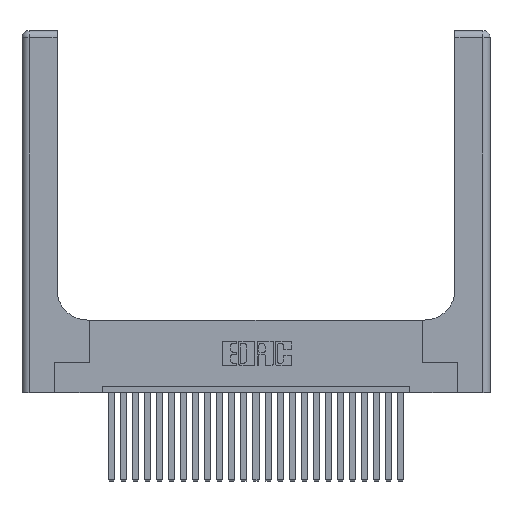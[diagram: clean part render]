
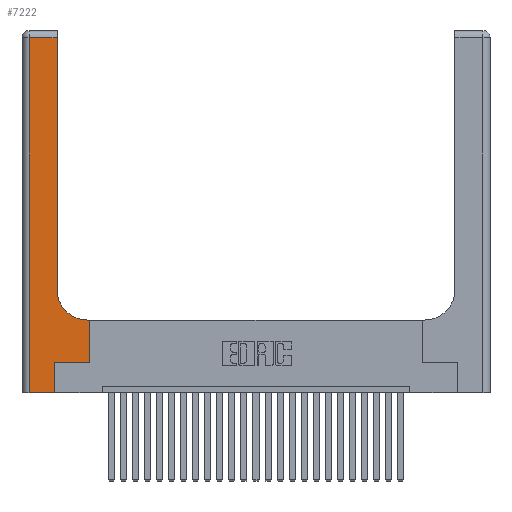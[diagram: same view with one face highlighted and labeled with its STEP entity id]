
A CAD part, top view. The second image highlights one B-rep face of the part: STEP entity #7222.
In plain terms, the highlighted planar face has unit normal (0, 0, 1).
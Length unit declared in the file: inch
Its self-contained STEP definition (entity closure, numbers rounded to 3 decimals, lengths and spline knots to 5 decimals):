
#53 = VERTEX_POINT ( 'NONE', #1612 ) ;
#74 = AXIS2_PLACEMENT_3D ( 'NONE', #4437, #18707, #6820 ) ;
#251 = CARTESIAN_POINT ( 'NONE',  ( 0.269, 0., 0.37 ) ) ;
#652 = VECTOR ( 'NONE', #22442, 39.37008 ) ;
#1354 = CARTESIAN_POINT ( 'NONE',  ( 0.269, 0.25, 0.37 ) ) ;
#1612 = CARTESIAN_POINT ( 'NONE',  ( 0.06, 2.94, 0.37 ) ) ;
#2027 = LINE ( 'NONE', #4778, #13988 ) ;
#2198 = DIRECTION ( 'NONE',  ( 0., 1., 0. ) ) ;
#2358 = VECTOR ( 'NONE', #20729, 39.37008 ) ;
#2909 = VERTEX_POINT ( 'NONE', #25321 ) ;
#2932 = LINE ( 'NONE', #18457, #23054 ) ;
#3047 = ORIENTED_EDGE ( 'NONE', *, *, #14848, .T. ) ;
#3260 = DIRECTION ( 'NONE',  ( 0., 0., -1. ) ) ;
#3556 = ORIENTED_EDGE ( 'NONE', *, *, #8674, .T. ) ;
#4031 = VERTEX_POINT ( 'NONE', #25972 ) ;
#4101 = ORIENTED_EDGE ( 'NONE', *, *, #18121, .T. ) ;
#4437 = CARTESIAN_POINT ( 'NONE',  ( 0.5415, 0.85, 0.37 ) ) ;
#4513 = ORIENTED_EDGE ( 'NONE', *, *, #19888, .T. ) ;
#4575 = ORIENTED_EDGE ( 'NONE', *, *, #22186, .T. ) ;
#4778 = CARTESIAN_POINT ( 'NONE',  ( 0.5585, 0.25, 0.37 ) ) ;
#4822 = CARTESIAN_POINT ( 'NONE',  ( 0.269, 0.25, 0.37 ) ) ;
#5112 = DIRECTION ( 'NONE',  ( -1., 0., 0. ) ) ;
#5388 = VERTEX_POINT ( 'NONE', #13021 ) ;
#5740 = ORIENTED_EDGE ( 'NONE', *, *, #19555, .T. ) ;
#5944 = CIRCLE ( 'NONE', #74, 0.25 ) ;
#6820 = DIRECTION ( 'NONE',  ( 1., 0., 0. ) ) ;
#6921 = LINE ( 'NONE', #251, #22953 ) ;
#7222 = ADVANCED_FACE ( 'NONE', ( #12793 ), #21305, .F. ) ;
#7678 = VERTEX_POINT ( 'NONE', #8028 ) ;
#8028 = CARTESIAN_POINT ( 'NONE',  ( 0.06, 0., 0.37 ) ) ;
#8210 = CARTESIAN_POINT ( 'NONE',  ( 0., 0., 0.37 ) ) ;
#8294 = LINE ( 'NONE', #1354, #20252 ) ;
#8306 = DIRECTION ( 'NONE',  ( 0., 1., 0. ) ) ;
#8623 = VERTEX_POINT ( 'NONE', #16592 ) ;
#8674 = EDGE_CURVE ( 'NONE', #15352, #53, #13393, .T. ) ;
#9237 = DIRECTION ( 'NONE',  ( 1., 0., 0. ) ) ;
#10196 = EDGE_CURVE ( 'NONE', #53, #7678, #2932, .T. ) ;
#11954 = AXIS2_PLACEMENT_3D ( 'NONE', #17180, #3260, #5112 ) ;
#12604 = CARTESIAN_POINT ( 'NONE',  ( 0., 2.94, 0.37 ) ) ;
#12760 = DIRECTION ( 'NONE',  ( 0., 1., 0. ) ) ;
#12793 = FACE_OUTER_BOUND ( 'NONE', #13052, .T. ) ;
#13021 = CARTESIAN_POINT ( 'NONE',  ( 0.269, 0., 0.37 ) ) ;
#13052 = EDGE_LOOP ( 'NONE', ( #14773, #3556, #19311, #4513, #3047, #18868, #4101, #5740, #4575 ) ) ;
#13393 = LINE ( 'NONE', #12604, #2358 ) ;
#13988 = VECTOR ( 'NONE', #12760, 39.37008 ) ;
#14025 = DIRECTION ( 'NONE',  ( 0., -1., 0. ) ) ;
#14773 = ORIENTED_EDGE ( 'NONE', *, *, #20964, .T. ) ;
#14848 = EDGE_CURVE ( 'NONE', #5388, #21677, #6921, .T. ) ;
#15171 = CARTESIAN_POINT ( 'NONE',  ( 0.2915, 0.6, 0.37 ) ) ;
#15352 = VERTEX_POINT ( 'NONE', #23555 ) ;
#15589 = VERTEX_POINT ( 'NONE', #18683 ) ;
#15806 = VECTOR ( 'NONE', #19149, 39.37008 ) ;
#16592 = CARTESIAN_POINT ( 'NONE',  ( 0.2915, 0.85, 0.37 ) ) ;
#17180 = CARTESIAN_POINT ( 'NONE',  ( 0., 3., 0.37 ) ) ;
#18121 = EDGE_CURVE ( 'NONE', #2909, #15589, #2027, .T. ) ;
#18284 = LINE ( 'NONE', #19812, #22967 ) ;
#18457 = CARTESIAN_POINT ( 'NONE',  ( 0.06, 3., 0.37 ) ) ;
#18683 = CARTESIAN_POINT ( 'NONE',  ( 0.5585, 0.6, 0.37 ) ) ;
#18707 = DIRECTION ( 'NONE',  ( 0., 0., -1. ) ) ;
#18868 = ORIENTED_EDGE ( 'NONE', *, *, #18967, .T. ) ;
#18967 = EDGE_CURVE ( 'NONE', #21677, #2909, #8294, .T. ) ;
#19149 = DIRECTION ( 'NONE',  ( -1., 0., 0. ) ) ;
#19272 = LINE ( 'NONE', #15171, #15806 ) ;
#19311 = ORIENTED_EDGE ( 'NONE', *, *, #10196, .T. ) ;
#19555 = EDGE_CURVE ( 'NONE', #15589, #4031, #19272, .T. ) ;
#19812 = CARTESIAN_POINT ( 'NONE',  ( 0.2915, 3., 0.37 ) ) ;
#19888 = EDGE_CURVE ( 'NONE', #7678, #5388, #22390, .T. ) ;
#20252 = VECTOR ( 'NONE', #9237, 39.37008 ) ;
#20729 = DIRECTION ( 'NONE',  ( -1., 0., 0. ) ) ;
#20964 = EDGE_CURVE ( 'NONE', #8623, #15352, #18284, .T. ) ;
#21305 = PLANE ( 'NONE',  #11954 ) ;
#21677 = VERTEX_POINT ( 'NONE', #4822 ) ;
#22186 = EDGE_CURVE ( 'NONE', #4031, #8623, #5944, .T. ) ;
#22390 = LINE ( 'NONE', #8210, #652 ) ;
#22442 = DIRECTION ( 'NONE',  ( 1., 0., 0. ) ) ;
#22953 = VECTOR ( 'NONE', #8306, 39.37008 ) ;
#22967 = VECTOR ( 'NONE', #2198, 39.37008 ) ;
#23054 = VECTOR ( 'NONE', #14025, 39.37008 ) ;
#23555 = CARTESIAN_POINT ( 'NONE',  ( 0.2915, 2.94, 0.37 ) ) ;
#25321 = CARTESIAN_POINT ( 'NONE',  ( 0.5585, 0.25, 0.37 ) ) ;
#25972 = CARTESIAN_POINT ( 'NONE',  ( 0.5415, 0.6, 0.37 ) ) ;
